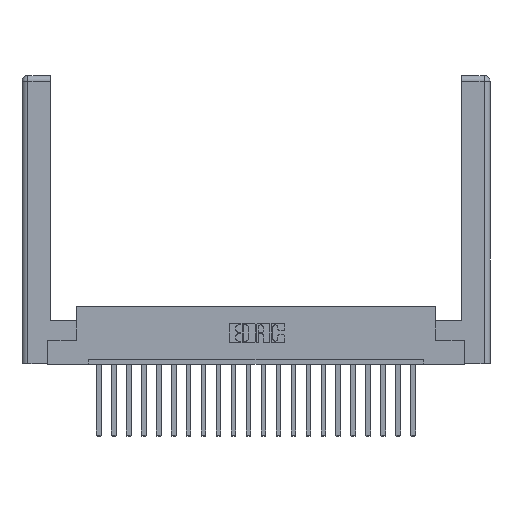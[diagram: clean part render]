
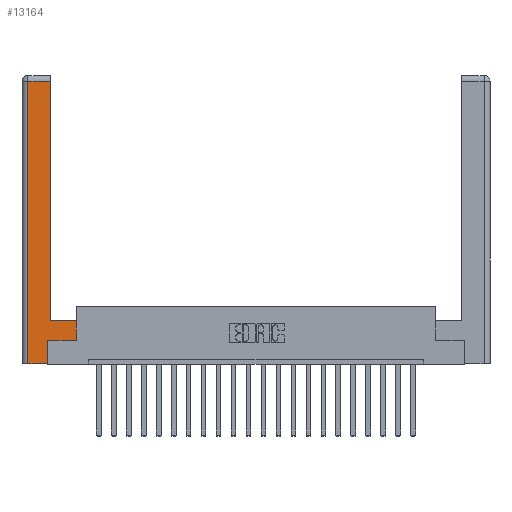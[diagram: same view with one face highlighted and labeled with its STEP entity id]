
A CAD part, top view. The second image highlights one B-rep face of the part: STEP entity #13164.
In plain terms, the highlighted planar face has unit normal (0, 0, 1).
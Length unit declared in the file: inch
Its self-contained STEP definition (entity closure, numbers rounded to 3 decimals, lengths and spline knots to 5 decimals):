
#936 = DIRECTION ( 'NONE',  ( -1., 0., 0. ) ) ;
#1066 = LINE ( 'NONE', #14863, #15772 ) ;
#1138 = EDGE_CURVE ( 'NONE', #14912, #17736, #16825, .T. ) ;
#2669 = VERTEX_POINT ( 'NONE', #8873 ) ;
#2830 = DIRECTION ( 'NONE',  ( 0., 0., -1. ) ) ;
#3169 = CARTESIAN_POINT ( 'NONE',  ( 0.0615, 0., 0. ) ) ;
#3308 = VECTOR ( 'NONE', #13210, 39.37008 ) ;
#3537 = CARTESIAN_POINT ( 'NONE',  ( 0.265, 0.245, 0. ) ) ;
#3613 = EDGE_LOOP ( 'NONE', ( #10998, #11846, #4590, #20571, #9462, #7146, #11031, #20066 ) ) ;
#4426 = LINE ( 'NONE', #3169, #11610 ) ;
#4440 = CARTESIAN_POINT ( 'NONE',  ( 0., 0., 0. ) ) ;
#4521 = VERTEX_POINT ( 'NONE', #5141 ) ;
#4590 = ORIENTED_EDGE ( 'NONE', *, *, #13544, .T. ) ;
#4815 = CARTESIAN_POINT ( 'NONE',  ( 0.0615, 0., 0. ) ) ;
#5141 = CARTESIAN_POINT ( 'NONE',  ( 0.565, 0.245, 0. ) ) ;
#5386 = LINE ( 'NONE', #14410, #11311 ) ;
#5647 = LINE ( 'NONE', #3537, #3308 ) ;
#5991 = FACE_OUTER_BOUND ( 'NONE', #3613, .T. ) ;
#5996 = CARTESIAN_POINT ( 'NONE',  ( 0.0615, 2.94, 0. ) ) ;
#6141 = VERTEX_POINT ( 'NONE', #14106 ) ;
#6806 = CARTESIAN_POINT ( 'NONE',  ( 0.265, 0., 0. ) ) ;
#7028 = LINE ( 'NONE', #9480, #10615 ) ;
#7059 = VECTOR ( 'NONE', #15877, 39.37008 ) ;
#7146 = ORIENTED_EDGE ( 'NONE', *, *, #9179, .T. ) ;
#8045 = DIRECTION ( 'NONE',  ( 0., 1., 0. ) ) ;
#8367 = EDGE_CURVE ( 'NONE', #18730, #2669, #12671, .T. ) ;
#8873 = CARTESIAN_POINT ( 'NONE',  ( 0.0615, 2.94, 0. ) ) ;
#9058 = EDGE_CURVE ( 'NONE', #17736, #6141, #5647, .T. ) ;
#9179 = EDGE_CURVE ( 'NONE', #6141, #4521, #5386, .T. ) ;
#9402 = PLANE ( 'NONE',  #11427 ) ;
#9462 = ORIENTED_EDGE ( 'NONE', *, *, #9058, .T. ) ;
#9480 = CARTESIAN_POINT ( 'NONE',  ( 0.565, 0.45, 0. ) ) ;
#10615 = VECTOR ( 'NONE', #8045, 39.37008 ) ;
#10998 = ORIENTED_EDGE ( 'NONE', *, *, #15239, .T. ) ;
#11031 = ORIENTED_EDGE ( 'NONE', *, *, #13275, .T. ) ;
#11094 = VECTOR ( 'NONE', #936, 39.37008 ) ;
#11311 = VECTOR ( 'NONE', #12677, 39.37008 ) ;
#11427 = AXIS2_PLACEMENT_3D ( 'NONE', #4440, #2830, #14375 ) ;
#11610 = VECTOR ( 'NONE', #19544, 39.37008 ) ;
#11677 = DIRECTION ( 'NONE',  ( -1., 0., 0. ) ) ;
#11846 = ORIENTED_EDGE ( 'NONE', *, *, #8367, .T. ) ;
#12515 = VECTOR ( 'NONE', #19235, 39.37008 ) ;
#12671 = LINE ( 'NONE', #5996, #11094 ) ;
#12677 = DIRECTION ( 'NONE',  ( 1., 0., 0. ) ) ;
#13164 = ADVANCED_FACE ( 'NONE', ( #5991 ), #9402, .F. ) ;
#13210 = DIRECTION ( 'NONE',  ( 0., 1., 0. ) ) ;
#13275 = EDGE_CURVE ( 'NONE', #4521, #15070, #7028, .T. ) ;
#13298 = LINE ( 'NONE', #20905, #12515 ) ;
#13337 = EDGE_CURVE ( 'NONE', #15070, #20578, #1066, .T. ) ;
#13544 = EDGE_CURVE ( 'NONE', #2669, #14912, #4426, .T. ) ;
#14106 = CARTESIAN_POINT ( 'NONE',  ( 0.265, 0.245, 0. ) ) ;
#14375 = DIRECTION ( 'NONE',  ( -1., 0., 0. ) ) ;
#14410 = CARTESIAN_POINT ( 'NONE',  ( 0.565, 0.245, 0. ) ) ;
#14863 = CARTESIAN_POINT ( 'NONE',  ( 0.295, 0.45, 0. ) ) ;
#14912 = VERTEX_POINT ( 'NONE', #4815 ) ;
#15070 = VERTEX_POINT ( 'NONE', #15092 ) ;
#15092 = CARTESIAN_POINT ( 'NONE',  ( 0.565, 0.45, 0. ) ) ;
#15239 = EDGE_CURVE ( 'NONE', #20578, #18730, #13298, .T. ) ;
#15772 = VECTOR ( 'NONE', #11677, 39.37008 ) ;
#15877 = DIRECTION ( 'NONE',  ( 1., 0., 0. ) ) ;
#16157 = CARTESIAN_POINT ( 'NONE',  ( 0.265, 0., 0. ) ) ;
#16825 = LINE ( 'NONE', #16157, #7059 ) ;
#17114 = CARTESIAN_POINT ( 'NONE',  ( 0.295, 2.94, 0. ) ) ;
#17704 = CARTESIAN_POINT ( 'NONE',  ( 0.295, 0.45, 0. ) ) ;
#17736 = VERTEX_POINT ( 'NONE', #6806 ) ;
#18730 = VERTEX_POINT ( 'NONE', #17114 ) ;
#19235 = DIRECTION ( 'NONE',  ( 0., 1., 0. ) ) ;
#19544 = DIRECTION ( 'NONE',  ( 0., -1., 0. ) ) ;
#20066 = ORIENTED_EDGE ( 'NONE', *, *, #13337, .T. ) ;
#20571 = ORIENTED_EDGE ( 'NONE', *, *, #1138, .T. ) ;
#20578 = VERTEX_POINT ( 'NONE', #17704 ) ;
#20905 = CARTESIAN_POINT ( 'NONE',  ( 0.295, 3., 0. ) ) ;
